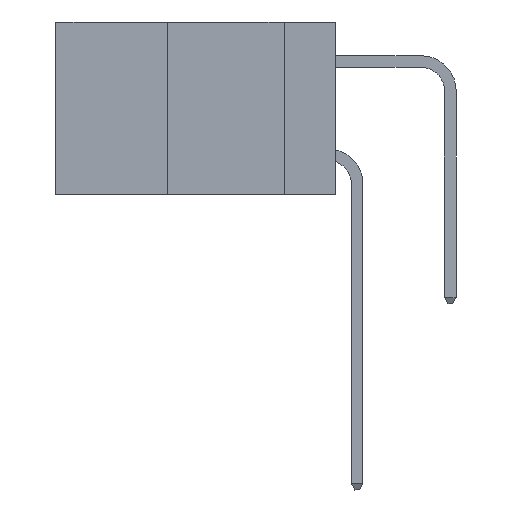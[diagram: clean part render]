
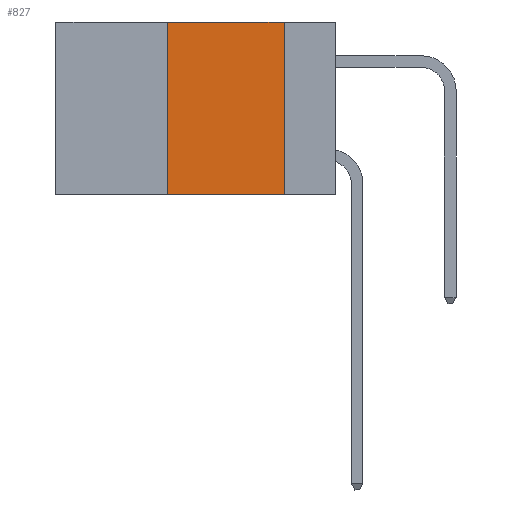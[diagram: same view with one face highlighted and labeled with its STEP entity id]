
A CAD part, left-side view. The second image highlights one B-rep face of the part: STEP entity #827.
In plain terms, the highlighted planar face has unit normal (-1, 0, 0).
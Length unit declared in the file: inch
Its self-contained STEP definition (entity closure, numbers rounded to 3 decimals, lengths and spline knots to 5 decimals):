
#274 = EDGE_LOOP ( 'NONE', ( #1538, #1850, #1606, #6107 ) ) ;
#778 = LINE ( 'NONE', #3812, #20112 ) ;
#827 = ADVANCED_FACE ( 'NONE', ( #23540 ), #6242, .F. ) ;
#1538 = ORIENTED_EDGE ( 'NONE', *, *, #7322, .F. ) ;
#1606 = ORIENTED_EDGE ( 'NONE', *, *, #6033, .F. ) ;
#1850 = ORIENTED_EDGE ( 'NONE', *, *, #9119, .F. ) ;
#2215 = VECTOR ( 'NONE', #23679, 39.37008 ) ;
#2278 = LINE ( 'NONE', #17927, #21603 ) ;
#2376 = VERTEX_POINT ( 'NONE', #19594 ) ;
#3812 = CARTESIAN_POINT ( 'NONE',  ( 0., 0.6, -0.37 ) ) ;
#3974 = CARTESIAN_POINT ( 'NONE',  ( 0., 0.36, 0. ) ) ;
#4478 = VERTEX_POINT ( 'NONE', #12271 ) ;
#5385 = CARTESIAN_POINT ( 'NONE',  ( 0., 0.6, 0. ) ) ;
#5511 = DIRECTION ( 'NONE',  ( 0., 0., -1. ) ) ;
#5768 = CARTESIAN_POINT ( 'NONE',  ( 0., 0.11, -0.37 ) ) ;
#5968 = VERTEX_POINT ( 'NONE', #5768 ) ;
#6033 = EDGE_CURVE ( 'NONE', #4478, #23068, #20444, .T. ) ;
#6107 = ORIENTED_EDGE ( 'NONE', *, *, #20246, .T. ) ;
#6242 = PLANE ( 'NONE',  #17225 ) ;
#7101 = DIRECTION ( 'NONE',  ( 1., 0., 0. ) ) ;
#7322 = EDGE_CURVE ( 'NONE', #2376, #5968, #11686, .T. ) ;
#7685 = DIRECTION ( 'NONE',  ( 0., -1., 0. ) ) ;
#9119 = EDGE_CURVE ( 'NONE', #23068, #2376, #2278, .T. ) ;
#9997 = VECTOR ( 'NONE', #15272, 39.37008 ) ;
#11686 = LINE ( 'NONE', #19954, #2215 ) ;
#12271 = CARTESIAN_POINT ( 'NONE',  ( 0., 0.36, -0.37 ) ) ;
#14937 = CARTESIAN_POINT ( 'NONE',  ( 0., 0.36, 0. ) ) ;
#15272 = DIRECTION ( 'NONE',  ( 0., 0., 1. ) ) ;
#16161 = DIRECTION ( 'NONE',  ( 0., -1., 0. ) ) ;
#17225 = AXIS2_PLACEMENT_3D ( 'NONE', #5385, #7101, #5511 ) ;
#17927 = CARTESIAN_POINT ( 'NONE',  ( 0., 0.6, 0. ) ) ;
#19594 = CARTESIAN_POINT ( 'NONE',  ( 0., 0.11, 0. ) ) ;
#19954 = CARTESIAN_POINT ( 'NONE',  ( 0., 0.11, 0. ) ) ;
#20112 = VECTOR ( 'NONE', #7685, 39.37008 ) ;
#20246 = EDGE_CURVE ( 'NONE', #4478, #5968, #778, .T. ) ;
#20444 = LINE ( 'NONE', #3974, #9997 ) ;
#21603 = VECTOR ( 'NONE', #16161, 39.37008 ) ;
#23068 = VERTEX_POINT ( 'NONE', #14937 ) ;
#23540 = FACE_OUTER_BOUND ( 'NONE', #274, .T. ) ;
#23679 = DIRECTION ( 'NONE',  ( 0., 0., -1. ) ) ;
